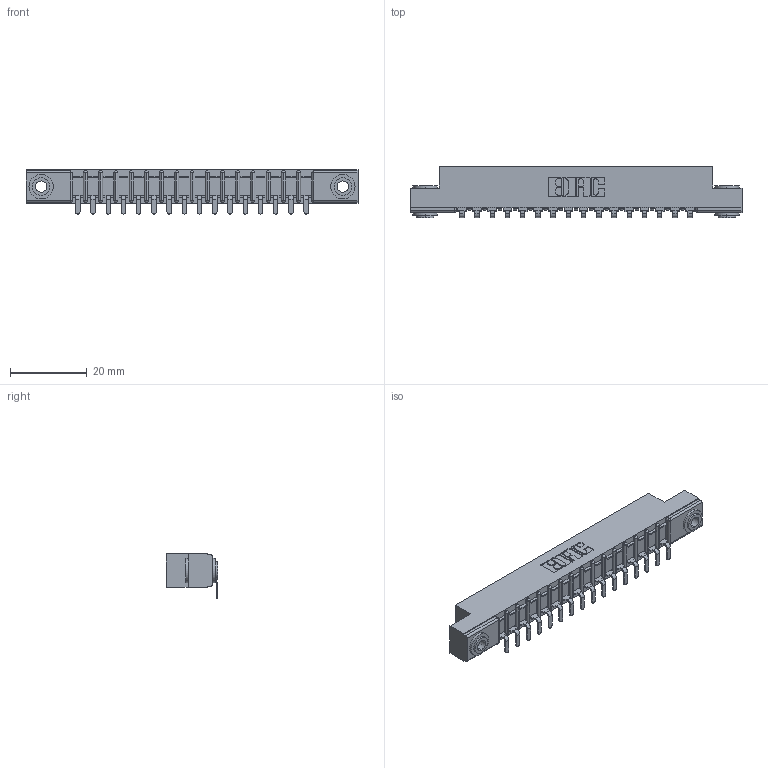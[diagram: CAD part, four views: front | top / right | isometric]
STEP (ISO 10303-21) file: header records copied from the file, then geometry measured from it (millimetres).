
FILE_DESCRIPTION (( 'STEP AP203' ), '1' );
FILE_NAME ('307-016-553-103.STEP', '2019-09-04T21:26:00', ( '' ), ( '' ), 'SwSTEP 2.0', 'SolidWorks 2016', '' );
FILE_SCHEMA (( 'CONFIG_CONTROL_DESIGN' ));
Length unit declared in the file: inch
Products named in the file (4): 307-016-553-103; 345-250-002_345-250-002-102; 307 Part_.156 Dia Mounting Holes; 307-290-002_553
Assembly tree (19 placements, depth 2):
  307-016-553-103
    307 Part_.156 Dia Mounting Holes
    307-290-002_553  x16
    345-250-002_345-250-002-102  x2
Bounding box: 86.41 x 13.36 x 11.51 mm (x, y, z)
Volume: 5702.8 mm3; surface area: 10287.5 mm2
Topology: 19 solids, 19 shells, 1435 faces, 4339 edges, 2842 vertices
Faces by surface type: plane 846, cylinder 547, sphere 34, cone 8
Entity records: 18841 total; most frequent: CARTESIAN_POINT 3153, ORIENTED_EDGE 3134, DIRECTION 3091, EDGE_CURVE 1567, VECTOR 1179, LINE 1179, VERTEX_POINT 1018, AXIS2_PLACEMENT_3D 956
